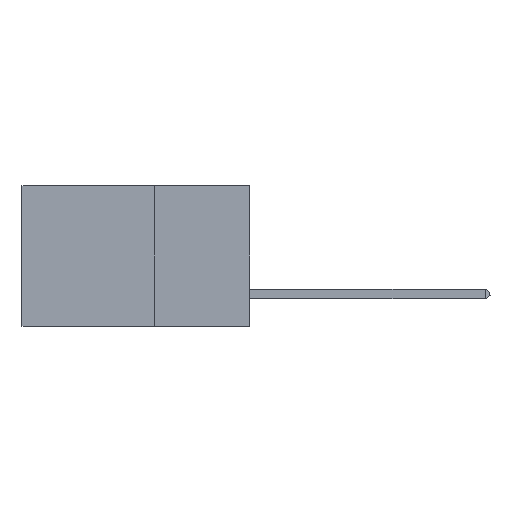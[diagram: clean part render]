
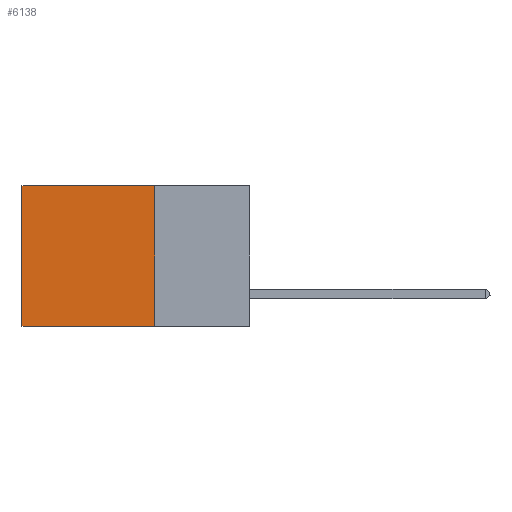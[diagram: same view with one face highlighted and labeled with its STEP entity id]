
A CAD part, left-side view. The second image highlights one B-rep face of the part: STEP entity #6138.
In plain terms, the highlighted planar face has unit normal (-1, 0, 0).
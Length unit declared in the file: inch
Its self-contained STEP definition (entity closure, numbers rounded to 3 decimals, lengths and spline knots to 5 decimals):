
#841 = DIRECTION ( 'NONE',  ( 0., 1., 0. ) ) ;
#1222 = DIRECTION ( 'NONE',  ( 0., 0., -1. ) ) ;
#1381 = VECTOR ( 'NONE', #841, 39.37008 ) ;
#1527 = VECTOR ( 'NONE', #1222, 39.37008 ) ;
#2303 = LINE ( 'NONE', #10233, #10537 ) ;
#2682 = LINE ( 'NONE', #6004, #6463 ) ;
#2942 = VERTEX_POINT ( 'NONE', #6866 ) ;
#3557 = EDGE_CURVE ( 'NONE', #2942, #10610, #2682, .T. ) ;
#3582 = PLANE ( 'NONE',  #7555 ) ;
#4078 = ORIENTED_EDGE ( 'NONE', *, *, #6820, .F. ) ;
#4203 = LINE ( 'NONE', #12270, #1527 ) ;
#5426 = ORIENTED_EDGE ( 'NONE', *, *, #3557, .T. ) ;
#5505 = FACE_OUTER_BOUND ( 'NONE', #12156, .T. ) ;
#5660 = LINE ( 'NONE', #10006, #1381 ) ;
#5791 = DIRECTION ( 'NONE',  ( 0., 0., -1. ) ) ;
#6004 = CARTESIAN_POINT ( 'NONE',  ( 0.2875, 0.25, 0. ) ) ;
#6138 = ADVANCED_FACE ( 'NONE', ( #5505 ), #3582, .F. ) ;
#6288 = ORIENTED_EDGE ( 'NONE', *, *, #11032, .T. ) ;
#6463 = VECTOR ( 'NONE', #11862, 39.37008 ) ;
#6820 = EDGE_CURVE ( 'NONE', #7384, #11363, #5660, .T. ) ;
#6866 = CARTESIAN_POINT ( 'NONE',  ( 0.2875, 0.25, 0. ) ) ;
#6883 = ORIENTED_EDGE ( 'NONE', *, *, #11239, .F. ) ;
#7384 = VERTEX_POINT ( 'NONE', #12667 ) ;
#7555 = AXIS2_PLACEMENT_3D ( 'NONE', #12847, #11844, #5791 ) ;
#9470 = CARTESIAN_POINT ( 'NONE',  ( 0.2875, 0.6, -0.37 ) ) ;
#10006 = CARTESIAN_POINT ( 'NONE',  ( 0.2875, 0.25, -0.37 ) ) ;
#10233 = CARTESIAN_POINT ( 'NONE',  ( 0.2875, 0.6, 0. ) ) ;
#10537 = VECTOR ( 'NONE', #11096, 39.37008 ) ;
#10610 = VERTEX_POINT ( 'NONE', #12407 ) ;
#11032 = EDGE_CURVE ( 'NONE', #10610, #11363, #2303, .T. ) ;
#11096 = DIRECTION ( 'NONE',  ( 0., 0., -1. ) ) ;
#11239 = EDGE_CURVE ( 'NONE', #2942, #7384, #4203, .T. ) ;
#11363 = VERTEX_POINT ( 'NONE', #9470 ) ;
#11844 = DIRECTION ( 'NONE',  ( 1., 0., 0. ) ) ;
#11862 = DIRECTION ( 'NONE',  ( 0., 1., 0. ) ) ;
#12156 = EDGE_LOOP ( 'NONE', ( #6288, #4078, #6883, #5426 ) ) ;
#12270 = CARTESIAN_POINT ( 'NONE',  ( 0.2875, 0.25, 0. ) ) ;
#12407 = CARTESIAN_POINT ( 'NONE',  ( 0.2875, 0.6, 0. ) ) ;
#12667 = CARTESIAN_POINT ( 'NONE',  ( 0.2875, 0.25, -0.37 ) ) ;
#12847 = CARTESIAN_POINT ( 'NONE',  ( 0.2875, 0.25, 0. ) ) ;
